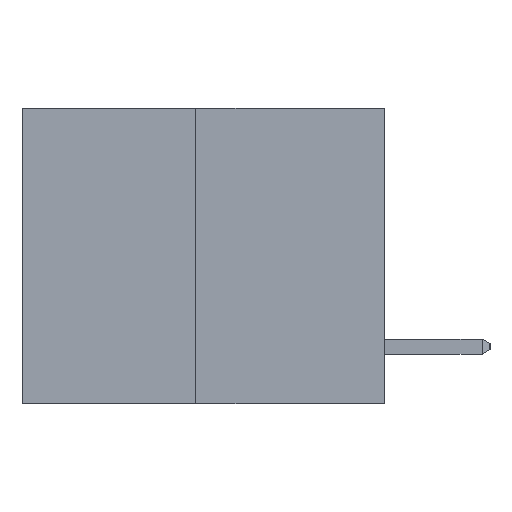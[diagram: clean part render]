
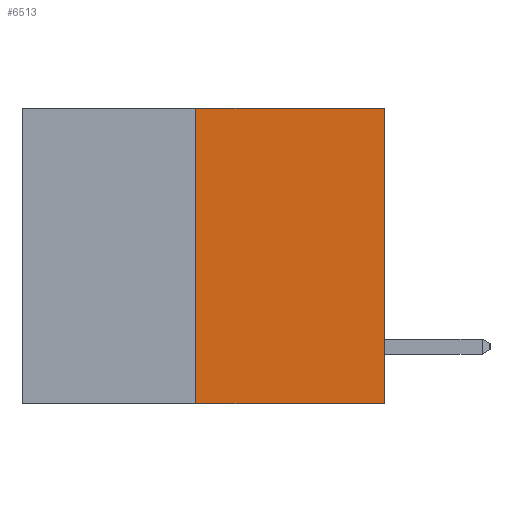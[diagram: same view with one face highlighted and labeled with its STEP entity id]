
A CAD part, left-side view. The second image highlights one B-rep face of the part: STEP entity #6513.
In plain terms, the highlighted planar face has unit normal (-1, 0, 0).
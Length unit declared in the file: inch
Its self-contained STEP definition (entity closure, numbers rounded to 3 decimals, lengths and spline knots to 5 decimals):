
#655 = VERTEX_POINT ( 'NONE', #15651 ) ;
#1144 = EDGE_CURVE ( 'NONE', #655, #2856, #13068, .T. ) ;
#1498 = VECTOR ( 'NONE', #16259, 39.37008 ) ;
#2082 = FACE_OUTER_BOUND ( 'NONE', #4604, .T. ) ;
#2856 = VERTEX_POINT ( 'NONE', #17486 ) ;
#2996 = CARTESIAN_POINT ( 'NONE',  ( 0., 0.6, 0. ) ) ;
#3206 = AXIS2_PLACEMENT_3D ( 'NONE', #2996, #12449, #10606 ) ;
#3452 = VERTEX_POINT ( 'NONE', #8295 ) ;
#4541 = VERTEX_POINT ( 'NONE', #7708 ) ;
#4604 = EDGE_LOOP ( 'NONE', ( #15156, #10818, #17691, #13915 ) ) ;
#4871 = LINE ( 'NONE', #8425, #1498 ) ;
#6513 = ADVANCED_FACE ( 'NONE', ( #2082 ), #13999, .F. ) ;
#6666 = CARTESIAN_POINT ( 'NONE',  ( 0., 0., 0. ) ) ;
#6694 = VECTOR ( 'NONE', #9808, 39.37008 ) ;
#7573 = DIRECTION ( 'NONE',  ( 0., 0., 1. ) ) ;
#7708 = CARTESIAN_POINT ( 'NONE',  ( 0., 0., 0. ) ) ;
#8295 = CARTESIAN_POINT ( 'NONE',  ( 0., 0.312, 0. ) ) ;
#8425 = CARTESIAN_POINT ( 'NONE',  ( 0., 0.6, 0. ) ) ;
#8450 = VECTOR ( 'NONE', #7573, 39.37008 ) ;
#9808 = DIRECTION ( 'NONE',  ( 0., 0., 1. ) ) ;
#9861 = LINE ( 'NONE', #6666, #6694 ) ;
#9969 = DIRECTION ( 'NONE',  ( 0., -1., 0. ) ) ;
#10496 = EDGE_CURVE ( 'NONE', #655, #3452, #12628, .T. ) ;
#10606 = DIRECTION ( 'NONE',  ( 0., 0., -1. ) ) ;
#10818 = ORIENTED_EDGE ( 'NONE', *, *, #1144, .T. ) ;
#11287 = EDGE_CURVE ( 'NONE', #2856, #4541, #9861, .T. ) ;
#11789 = CARTESIAN_POINT ( 'NONE',  ( 0., 0.6, -0.49 ) ) ;
#12449 = DIRECTION ( 'NONE',  ( 1., 0., 0. ) ) ;
#12628 = LINE ( 'NONE', #15393, #8450 ) ;
#13068 = LINE ( 'NONE', #11789, #16710 ) ;
#13915 = ORIENTED_EDGE ( 'NONE', *, *, #19426, .F. ) ;
#13999 = PLANE ( 'NONE',  #3206 ) ;
#15156 = ORIENTED_EDGE ( 'NONE', *, *, #10496, .F. ) ;
#15393 = CARTESIAN_POINT ( 'NONE',  ( 0., 0.312, -0.49 ) ) ;
#15651 = CARTESIAN_POINT ( 'NONE',  ( 0., 0.312, -0.49 ) ) ;
#16259 = DIRECTION ( 'NONE',  ( 0., -1., 0. ) ) ;
#16710 = VECTOR ( 'NONE', #9969, 39.37008 ) ;
#17486 = CARTESIAN_POINT ( 'NONE',  ( 0., 0., -0.49 ) ) ;
#17691 = ORIENTED_EDGE ( 'NONE', *, *, #11287, .T. ) ;
#19426 = EDGE_CURVE ( 'NONE', #3452, #4541, #4871, .T. ) ;
